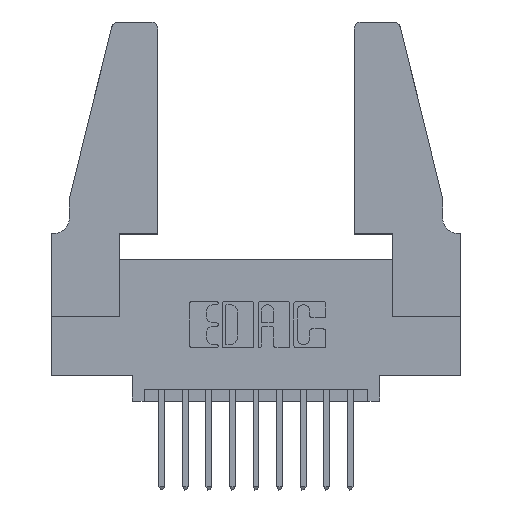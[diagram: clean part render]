
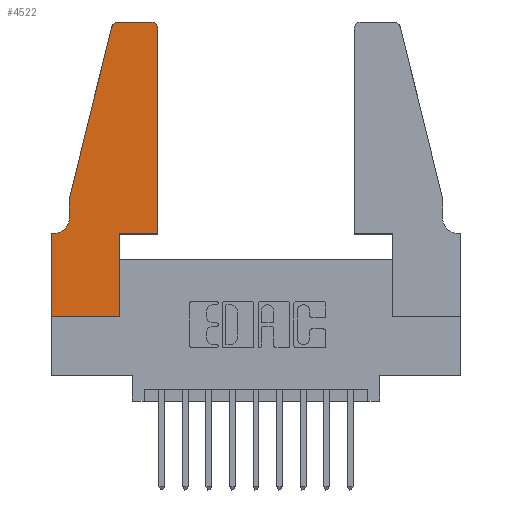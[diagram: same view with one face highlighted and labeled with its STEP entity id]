
A CAD part, top view. The second image highlights one B-rep face of the part: STEP entity #4522.
In plain terms, the highlighted planar face has unit normal (0, 0, 1).
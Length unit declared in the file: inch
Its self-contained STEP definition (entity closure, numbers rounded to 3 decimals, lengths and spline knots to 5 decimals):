
#173 = ORIENTED_EDGE ( 'NONE', *, *, #13506, .T. ) ;
#253 = AXIS2_PLACEMENT_3D ( 'NONE', #282, #1173, #10790 ) ;
#282 = CARTESIAN_POINT ( 'NONE',  ( 0.4205, 1.22, 0.37 ) ) ;
#556 = ORIENTED_EDGE ( 'NONE', *, *, #5554, .T. ) ;
#583 = LINE ( 'NONE', #9214, #7073 ) ;
#672 = CARTESIAN_POINT ( 'NONE',  ( 0.25487, 1.22718, 0.37 ) ) ;
#682 = CARTESIAN_POINT ( 'NONE',  ( 0.2865, 0.35, 0.37 ) ) ;
#683 = VECTOR ( 'NONE', #13427, 39.37008 ) ;
#697 = DIRECTION ( 'NONE',  ( 0., 0., 1. ) ) ;
#699 = LINE ( 'NONE', #10194, #12193 ) ;
#826 = LINE ( 'NONE', #1107, #1823 ) ;
#938 = VERTEX_POINT ( 'NONE', #13770 ) ;
#990 = VERTEX_POINT ( 'NONE', #6366 ) ;
#1107 = CARTESIAN_POINT ( 'NONE',  ( 0.4505, 0.35, 0.37 ) ) ;
#1173 = DIRECTION ( 'NONE',  ( 0., 0., 1. ) ) ;
#1509 = EDGE_CURVE ( 'NONE', #2894, #3256, #699, .T. ) ;
#1663 = ORIENTED_EDGE ( 'NONE', *, *, #10096, .T. ) ;
#1815 = VERTEX_POINT ( 'NONE', #12561 ) ;
#1823 = VECTOR ( 'NONE', #10641, 39.37008 ) ;
#1873 = EDGE_CURVE ( 'NONE', #2625, #938, #6326, .T. ) ;
#1903 = CARTESIAN_POINT ( 'NONE',  ( 0.0755, 0.42, 0.37 ) ) ;
#2190 = CARTESIAN_POINT ( 'NONE',  ( 0.4205, 1.25, 0.37 ) ) ;
#2194 = EDGE_CURVE ( 'NONE', #12379, #13455, #7810, .T. ) ;
#2238 = VERTEX_POINT ( 'NONE', #2190 ) ;
#2435 = CARTESIAN_POINT ( 'NONE',  ( 0., 0.35, 0.37 ) ) ;
#2561 = ORIENTED_EDGE ( 'NONE', *, *, #7414, .T. ) ;
#2625 = VERTEX_POINT ( 'NONE', #8457 ) ;
#2642 = CARTESIAN_POINT ( 'NONE',  ( 0.0755, 0.35, 0.37 ) ) ;
#2803 = EDGE_CURVE ( 'NONE', #938, #990, #826, .T. ) ;
#2894 = VERTEX_POINT ( 'NONE', #5691 ) ;
#3031 = ORIENTED_EDGE ( 'NONE', *, *, #8643, .T. ) ;
#3189 = CARTESIAN_POINT ( 'NONE',  ( 0.0755, 0.5, 0.37 ) ) ;
#3256 = VERTEX_POINT ( 'NONE', #12936 ) ;
#3582 = CIRCLE ( 'NONE', #253, 0.03 ) ;
#3630 = DIRECTION ( 'NONE',  ( 1., 0., 0. ) ) ;
#3872 = DIRECTION ( 'NONE',  ( -1., 0., 0. ) ) ;
#4291 = DIRECTION ( 'NONE',  ( 0., 0., 1. ) ) ;
#4452 = VECTOR ( 'NONE', #10261, 39.37008 ) ;
#4518 = AXIS2_PLACEMENT_3D ( 'NONE', #9394, #4291, #6522 ) ;
#4522 = ADVANCED_FACE ( 'NONE', ( #11604 ), #9350, .T. ) ;
#4737 = VECTOR ( 'NONE', #11076, 39.37008 ) ;
#5020 = DIRECTION ( 'NONE',  ( 1., 0., 0. ) ) ;
#5045 = CARTESIAN_POINT ( 'NONE',  ( 0.0055, 0.42, 0.37 ) ) ;
#5260 = VECTOR ( 'NONE', #11240, 39.37008 ) ;
#5297 = CARTESIAN_POINT ( 'NONE',  ( 0.284, 1.25, 0.37 ) ) ;
#5414 = EDGE_CURVE ( 'NONE', #990, #2238, #3582, .T. ) ;
#5554 = EDGE_CURVE ( 'NONE', #1815, #12111, #8885, .T. ) ;
#5691 = CARTESIAN_POINT ( 'NONE',  ( 0., 0., 0.37 ) ) ;
#6326 = LINE ( 'NONE', #8150, #683 ) ;
#6340 = VECTOR ( 'NONE', #13726, 39.37008 ) ;
#6366 = CARTESIAN_POINT ( 'NONE',  ( 0.4505, 1.22, 0.37 ) ) ;
#6506 = ORIENTED_EDGE ( 'NONE', *, *, #1509, .T. ) ;
#6522 = DIRECTION ( 'NONE',  ( 1., 0., 0. ) ) ;
#6877 = ORIENTED_EDGE ( 'NONE', *, *, #5414, .T. ) ;
#7002 = DIRECTION ( 'NONE',  ( -1., 0., 0. ) ) ;
#7051 = DIRECTION ( 'NONE',  ( 0., 0., -1. ) ) ;
#7073 = VECTOR ( 'NONE', #3872, 39.37008 ) ;
#7171 = ORIENTED_EDGE ( 'NONE', *, *, #2194, .T. ) ;
#7414 = EDGE_CURVE ( 'NONE', #3256, #2625, #11466, .T. ) ;
#7750 = LINE ( 'NONE', #2642, #5260 ) ;
#7810 = CIRCLE ( 'NONE', #9834, 0.03 ) ;
#8146 = ORIENTED_EDGE ( 'NONE', *, *, #8621, .T. ) ;
#8150 = CARTESIAN_POINT ( 'NONE',  ( 0.4505, 0.35, 0.37 ) ) ;
#8152 = CARTESIAN_POINT ( 'NONE',  ( 0.284, 1.22, 0.37 ) ) ;
#8457 = CARTESIAN_POINT ( 'NONE',  ( 0.2865, 0.35, 0.37 ) ) ;
#8607 = DIRECTION ( 'NONE',  ( -0.239, -0.971, 0. ) ) ;
#8621 = EDGE_CURVE ( 'NONE', #2238, #12379, #583, .T. ) ;
#8643 = EDGE_CURVE ( 'NONE', #12111, #11477, #13287, .T. ) ;
#8885 = LINE ( 'NONE', #10095, #4737 ) ;
#9172 = EDGE_LOOP ( 'NONE', ( #8146, #7171, #1663, #556, #3031, #173, #13013, #6506, #2561, #9831, #9937, #6877 ) ) ;
#9179 = AXIS2_PLACEMENT_3D ( 'NONE', #5045, #7051, #7002 ) ;
#9214 = CARTESIAN_POINT ( 'NONE',  ( 0.2605, 1.25, 0.37 ) ) ;
#9301 = CARTESIAN_POINT ( 'NONE',  ( 0., 0., 0.37 ) ) ;
#9350 = PLANE ( 'NONE',  #4518 ) ;
#9394 = CARTESIAN_POINT ( 'NONE',  ( 0., 0.35, 0.37 ) ) ;
#9831 = ORIENTED_EDGE ( 'NONE', *, *, #1873, .T. ) ;
#9834 = AXIS2_PLACEMENT_3D ( 'NONE', #8152, #697, #5020 ) ;
#9937 = ORIENTED_EDGE ( 'NONE', *, *, #2803, .T. ) ;
#10095 = CARTESIAN_POINT ( 'NONE',  ( 0.0755, 0.5, 0.37 ) ) ;
#10096 = EDGE_CURVE ( 'NONE', #13455, #1815, #12050, .T. ) ;
#10194 = CARTESIAN_POINT ( 'NONE',  ( 0., 0., 0.37 ) ) ;
#10261 = DIRECTION ( 'NONE',  ( 0., 1., 0. ) ) ;
#10641 = DIRECTION ( 'NONE',  ( 0., 1., 0. ) ) ;
#10701 = EDGE_CURVE ( 'NONE', #11846, #2894, #13227, .T. ) ;
#10790 = DIRECTION ( 'NONE',  ( 1., 0., 0. ) ) ;
#11076 = DIRECTION ( 'NONE',  ( 0., -1., 0. ) ) ;
#11240 = DIRECTION ( 'NONE',  ( -1., 0., 0. ) ) ;
#11466 = LINE ( 'NONE', #682, #4452 ) ;
#11477 = VERTEX_POINT ( 'NONE', #13240 ) ;
#11604 = FACE_OUTER_BOUND ( 'NONE', #9172, .T. ) ;
#11846 = VERTEX_POINT ( 'NONE', #2435 ) ;
#12050 = LINE ( 'NONE', #3189, #13076 ) ;
#12111 = VERTEX_POINT ( 'NONE', #1903 ) ;
#12193 = VECTOR ( 'NONE', #3630, 39.37008 ) ;
#12379 = VERTEX_POINT ( 'NONE', #5297 ) ;
#12561 = CARTESIAN_POINT ( 'NONE',  ( 0.0755, 0.5, 0.37 ) ) ;
#12936 = CARTESIAN_POINT ( 'NONE',  ( 0.2865, 0., 0.37 ) ) ;
#13013 = ORIENTED_EDGE ( 'NONE', *, *, #10701, .T. ) ;
#13076 = VECTOR ( 'NONE', #8607, 39.37008 ) ;
#13227 = LINE ( 'NONE', #9301, #6340 ) ;
#13240 = CARTESIAN_POINT ( 'NONE',  ( 0.0055, 0.35, 0.37 ) ) ;
#13287 = CIRCLE ( 'NONE', #9179, 0.07 ) ;
#13427 = DIRECTION ( 'NONE',  ( 1., 0., 0. ) ) ;
#13455 = VERTEX_POINT ( 'NONE', #672 ) ;
#13506 = EDGE_CURVE ( 'NONE', #11477, #11846, #7750, .T. ) ;
#13726 = DIRECTION ( 'NONE',  ( 0., -1., 0. ) ) ;
#13770 = CARTESIAN_POINT ( 'NONE',  ( 0.4505, 0.35, 0.37 ) ) ;
